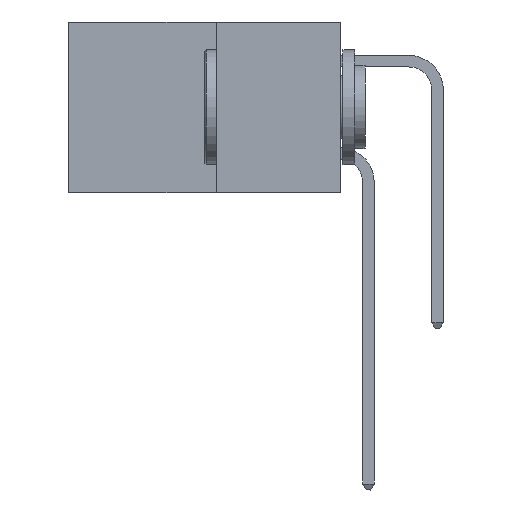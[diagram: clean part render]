
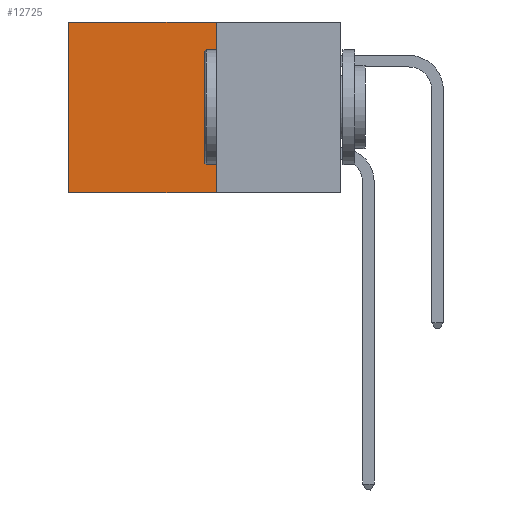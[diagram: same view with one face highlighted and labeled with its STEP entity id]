
A CAD part, left-side view. The second image highlights one B-rep face of the part: STEP entity #12725.
In plain terms, the highlighted planar face has unit normal (-1, 0, 0).
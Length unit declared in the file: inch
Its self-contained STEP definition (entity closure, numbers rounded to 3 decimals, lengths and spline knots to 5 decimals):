
#33 = DIRECTION ( 'NONE',  ( 0., 0., -1. ) ) ;
#579 = CARTESIAN_POINT ( 'NONE',  ( 0.277, 0.59, 0. ) ) ;
#761 = EDGE_LOOP ( 'NONE', ( #2026, #19860, #16608, #20868 ) ) ;
#1297 = DIRECTION ( 'NONE',  ( 1., 0., 0. ) ) ;
#1727 = EDGE_CURVE ( 'NONE', #11663, #7337, #2395, .T. ) ;
#2026 = ORIENTED_EDGE ( 'NONE', *, *, #1727, .T. ) ;
#2395 = LINE ( 'NONE', #4778, #14944 ) ;
#2403 = DIRECTION ( 'NONE',  ( 0., 1., 0. ) ) ;
#2558 = DIRECTION ( 'NONE',  ( 0., 0., -1. ) ) ;
#3607 = VERTEX_POINT ( 'NONE', #19187 ) ;
#3670 = LINE ( 'NONE', #10680, #7542 ) ;
#4607 = CARTESIAN_POINT ( 'NONE',  ( 0.277, 0.27, 0. ) ) ;
#4778 = CARTESIAN_POINT ( 'NONE',  ( 0.277, 0.59, -0.37 ) ) ;
#7205 = DIRECTION ( 'NONE',  ( 0., 0., -1. ) ) ;
#7337 = VERTEX_POINT ( 'NONE', #11667 ) ;
#7510 = AXIS2_PLACEMENT_3D ( 'NONE', #11097, #1297, #33 ) ;
#7542 = VECTOR ( 'NONE', #2558, 39.37008 ) ;
#7792 = CARTESIAN_POINT ( 'NONE',  ( 0.277, 0.27, -0.37 ) ) ;
#10094 = VECTOR ( 'NONE', #12679, 39.37008 ) ;
#10680 = CARTESIAN_POINT ( 'NONE',  ( 0.277, 0.27, -0.37 ) ) ;
#11097 = CARTESIAN_POINT ( 'NONE',  ( 0.277, 0.27, -0.37 ) ) ;
#11641 = VECTOR ( 'NONE', #2403, 39.37008 ) ;
#11663 = VERTEX_POINT ( 'NONE', #579 ) ;
#11667 = CARTESIAN_POINT ( 'NONE',  ( 0.277, 0.59, -0.37 ) ) ;
#12214 = CARTESIAN_POINT ( 'NONE',  ( 0.277, 0.27, 0. ) ) ;
#12679 = DIRECTION ( 'NONE',  ( 0., 1., 0. ) ) ;
#12725 = ADVANCED_FACE ( 'NONE', ( #13286 ), #20803, .F. ) ;
#13286 = FACE_OUTER_BOUND ( 'NONE', #761, .T. ) ;
#14498 = LINE ( 'NONE', #7792, #10094 ) ;
#14944 = VECTOR ( 'NONE', #7205, 39.37008 ) ;
#14972 = EDGE_CURVE ( 'NONE', #3607, #7337, #14498, .T. ) ;
#15988 = LINE ( 'NONE', #12214, #11641 ) ;
#16026 = EDGE_CURVE ( 'NONE', #16789, #11663, #15988, .T. ) ;
#16608 = ORIENTED_EDGE ( 'NONE', *, *, #18024, .F. ) ;
#16789 = VERTEX_POINT ( 'NONE', #4607 ) ;
#18024 = EDGE_CURVE ( 'NONE', #16789, #3607, #3670, .T. ) ;
#19187 = CARTESIAN_POINT ( 'NONE',  ( 0.277, 0.27, -0.37 ) ) ;
#19860 = ORIENTED_EDGE ( 'NONE', *, *, #14972, .F. ) ;
#20803 = PLANE ( 'NONE',  #7510 ) ;
#20868 = ORIENTED_EDGE ( 'NONE', *, *, #16026, .T. ) ;
